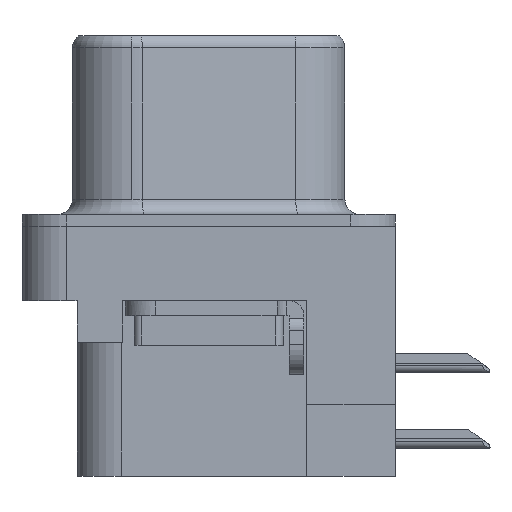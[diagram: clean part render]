
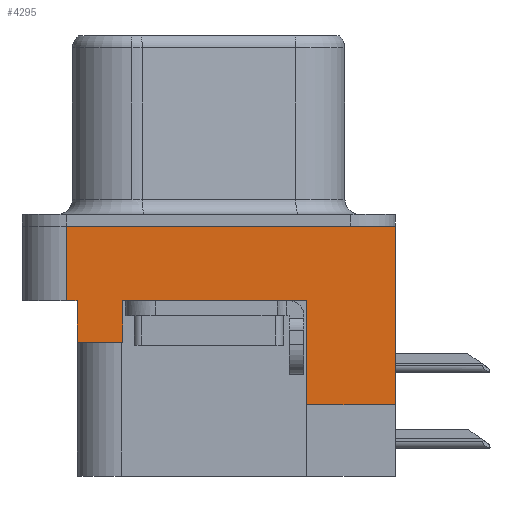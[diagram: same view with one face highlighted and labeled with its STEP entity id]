
A CAD part, left-side view. The second image highlights one B-rep face of the part: STEP entity #4295.
In plain terms, the highlighted planar face has unit normal (-1, 0, 0).
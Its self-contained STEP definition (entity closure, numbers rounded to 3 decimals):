
#434 = LINE ( 'NONE', #3659, #16202 ) ;
#449 = DIRECTION ( 'NONE',  ( 0., 0., 1. ) ) ;
#705 = CARTESIAN_POINT ( 'NONE',  ( -3., -6.275, -2.5 ) ) ;
#940 = VERTEX_POINT ( 'NONE', #7594 ) ;
#1275 = DIRECTION ( 'NONE',  ( 0., -1., 0. ) ) ;
#1621 = DIRECTION ( 'NONE',  ( 0., -1., 0. ) ) ;
#1929 = CARTESIAN_POINT ( 'NONE',  ( -3., 4.775, -2.5 ) ) ;
#2238 = VERTEX_POINT ( 'NONE', #5815 ) ;
#2380 = VERTEX_POINT ( 'NONE', #11262 ) ;
#2851 = LINE ( 'NONE', #705, #3089 ) ;
#3089 = VECTOR ( 'NONE', #9929, 1000. ) ;
#3325 = VECTOR ( 'NONE', #1621, 1000. ) ;
#3574 = LINE ( 'NONE', #15530, #3325 ) ;
#3659 = CARTESIAN_POINT ( 'NONE',  ( -3., -3.295, -8.4 ) ) ;
#4295 = ADVANCED_FACE ( 'NONE', ( #13189 ), #10169, .T. ) ;
#5075 = ORIENTED_EDGE ( 'NONE', *, *, #16427, .F. ) ;
#5077 = CARTESIAN_POINT ( 'NONE',  ( -3., -6.275, -6. ) ) ;
#5121 = CARTESIAN_POINT ( 'NONE',  ( -3., 4.425, -3.9 ) ) ;
#5144 = CARTESIAN_POINT ( 'NONE',  ( -3., -6.275, -2.5 ) ) ;
#5322 = VERTEX_POINT ( 'NONE', #7537 ) ;
#5652 = VERTEX_POINT ( 'NONE', #9319 ) ;
#5675 = ORIENTED_EDGE ( 'NONE', *, *, #17091, .T. ) ;
#5684 = CARTESIAN_POINT ( 'NONE',  ( -3., 2.895, -3.9 ) ) ;
#5815 = CARTESIAN_POINT ( 'NONE',  ( -3., 4.425, -3.9 ) ) ;
#5909 = ORIENTED_EDGE ( 'NONE', *, *, #17581, .F. ) ;
#5967 = EDGE_LOOP ( 'NONE', ( #11269, #5675, #5909, #18203, #8472, #17314, #5075, #16672, #10623, #12197 ) ) ;
#6785 = VECTOR ( 'NONE', #13691, 1000. ) ;
#7341 = CARTESIAN_POINT ( 'NONE',  ( -3., 4.775, 0. ) ) ;
#7416 = VERTEX_POINT ( 'NONE', #11092 ) ;
#7537 = CARTESIAN_POINT ( 'NONE',  ( -3., 4.775, -2.5 ) ) ;
#7594 = CARTESIAN_POINT ( 'NONE',  ( -3., -6.275, 0. ) ) ;
#7802 = LINE ( 'NONE', #14277, #11388 ) ;
#7955 = VERTEX_POINT ( 'NONE', #5077 ) ;
#8472 = ORIENTED_EDGE ( 'NONE', *, *, #16522, .T. ) ;
#8678 = DIRECTION ( 'NONE',  ( 0., 0., 1. ) ) ;
#8946 = CARTESIAN_POINT ( 'NONE',  ( -3., -6.275, 0. ) ) ;
#9132 = LINE ( 'NONE', #19914, #6785 ) ;
#9319 = CARTESIAN_POINT ( 'NONE',  ( -3., -3.295, -6. ) ) ;
#9929 = DIRECTION ( 'NONE',  ( 0., -1., 0. ) ) ;
#10169 = PLANE ( 'NONE',  #16535 ) ;
#10623 = ORIENTED_EDGE ( 'NONE', *, *, #16106, .T. ) ;
#11092 = CARTESIAN_POINT ( 'NONE',  ( -3., 2.895, -3.9 ) ) ;
#11262 = CARTESIAN_POINT ( 'NONE',  ( -3., 2.895, -2.5 ) ) ;
#11269 = ORIENTED_EDGE ( 'NONE', *, *, #17067, .F. ) ;
#11342 = DIRECTION ( 'NONE',  ( 0., 0., 1. ) ) ;
#11388 = VECTOR ( 'NONE', #15951, 1000. ) ;
#11559 = LINE ( 'NONE', #1929, #12473 ) ;
#12197 = ORIENTED_EDGE ( 'NONE', *, *, #18158, .F. ) ;
#12473 = VECTOR ( 'NONE', #15849, 1000. ) ;
#12515 = LINE ( 'NONE', #8946, #19821 ) ;
#13143 = CARTESIAN_POINT ( 'NONE',  ( -3., 4.425, -2.5 ) ) ;
#13178 = CARTESIAN_POINT ( 'NONE',  ( -3., -6.275, -2.5 ) ) ;
#13189 = FACE_OUTER_BOUND ( 'NONE', #5967, .T. ) ;
#13411 = LINE ( 'NONE', #5121, #15148 ) ;
#13691 = DIRECTION ( 'NONE',  ( 0., 1., 0. ) ) ;
#14161 = VERTEX_POINT ( 'NONE', #7341 ) ;
#14277 = CARTESIAN_POINT ( 'NONE',  ( -3., -6.495, -6. ) ) ;
#14380 = DIRECTION ( 'NONE',  ( 0., 0., 1. ) ) ;
#14570 = VERTEX_POINT ( 'NONE', #18800 ) ;
#14815 = DIRECTION ( 'NONE',  ( 0., 0., 1. ) ) ;
#15148 = VECTOR ( 'NONE', #449, 1000. ) ;
#15389 = VECTOR ( 'NONE', #14815, 1000. ) ;
#15530 = CARTESIAN_POINT ( 'NONE',  ( -3., -6.275, -2.5 ) ) ;
#15849 = DIRECTION ( 'NONE',  ( 0., 0., 1. ) ) ;
#15951 = DIRECTION ( 'NONE',  ( 0., 1., 0. ) ) ;
#15997 = LINE ( 'NONE', #5144, #18455 ) ;
#16106 = EDGE_CURVE ( 'NONE', #2380, #14570, #2851, .T. ) ;
#16202 = VECTOR ( 'NONE', #14380, 1000. ) ;
#16271 = EDGE_CURVE ( 'NONE', #7416, #2380, #17416, .T. ) ;
#16427 = EDGE_CURVE ( 'NONE', #7416, #2238, #9132, .T. ) ;
#16522 = EDGE_CURVE ( 'NONE', #5322, #16735, #3574, .T. ) ;
#16535 = AXIS2_PLACEMENT_3D ( 'NONE', #13178, #17986, #8678 ) ;
#16672 = ORIENTED_EDGE ( 'NONE', *, *, #16271, .T. ) ;
#16735 = VERTEX_POINT ( 'NONE', #13143 ) ;
#17067 = EDGE_CURVE ( 'NONE', #7955, #5652, #7802, .T. ) ;
#17091 = EDGE_CURVE ( 'NONE', #7955, #940, #15997, .T. ) ;
#17314 = ORIENTED_EDGE ( 'NONE', *, *, #18118, .F. ) ;
#17416 = LINE ( 'NONE', #5684, #15389 ) ;
#17581 = EDGE_CURVE ( 'NONE', #14161, #940, #12515, .T. ) ;
#17986 = DIRECTION ( 'NONE',  ( -1., 0., 0. ) ) ;
#18092 = EDGE_CURVE ( 'NONE', #5322, #14161, #11559, .T. ) ;
#18118 = EDGE_CURVE ( 'NONE', #2238, #16735, #13411, .T. ) ;
#18158 = EDGE_CURVE ( 'NONE', #5652, #14570, #434, .T. ) ;
#18203 = ORIENTED_EDGE ( 'NONE', *, *, #18092, .F. ) ;
#18455 = VECTOR ( 'NONE', #11342, 1000. ) ;
#18800 = CARTESIAN_POINT ( 'NONE',  ( -3., -3.295, -2.5 ) ) ;
#19821 = VECTOR ( 'NONE', #1275, 1000. ) ;
#19914 = CARTESIAN_POINT ( 'NONE',  ( -3., 4.425, -3.9 ) ) ;
